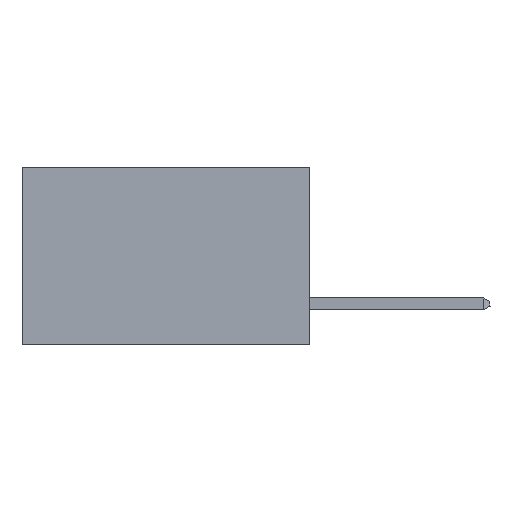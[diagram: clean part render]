
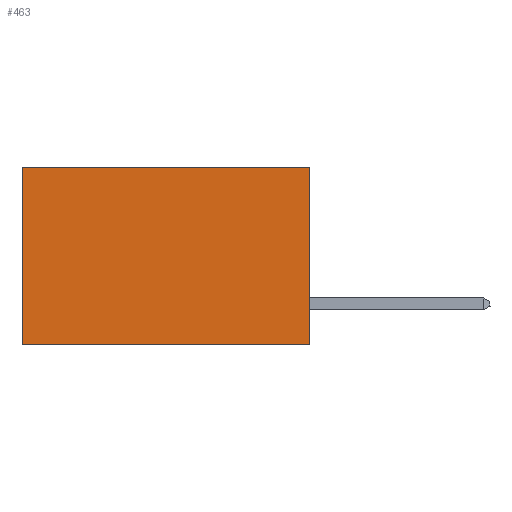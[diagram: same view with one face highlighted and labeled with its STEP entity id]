
A CAD part, left-side view. The second image highlights one B-rep face of the part: STEP entity #463.
In plain terms, the highlighted planar face has unit normal (-1, 0, 0).
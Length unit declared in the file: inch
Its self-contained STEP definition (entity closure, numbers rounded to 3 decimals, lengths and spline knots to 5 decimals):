
#463 = ADVANCED_FACE ( 'NONE', ( #3504 ), #22064, .F. ) ;
#1447 = CARTESIAN_POINT ( 'NONE',  ( 0.2875, 0., 0. ) ) ;
#1668 = ORIENTED_EDGE ( 'NONE', *, *, #17843, .T. ) ;
#1670 = LINE ( 'NONE', #1447, #18792 ) ;
#2592 = VERTEX_POINT ( 'NONE', #8639 ) ;
#2808 = LINE ( 'NONE', #9005, #14001 ) ;
#3261 = AXIS2_PLACEMENT_3D ( 'NONE', #5212, #9715, #4883 ) ;
#3504 = FACE_OUTER_BOUND ( 'NONE', #24174, .T. ) ;
#3709 = DIRECTION ( 'NONE',  ( 0., 0., -1. ) ) ;
#4883 = DIRECTION ( 'NONE',  ( 0., 0., -1. ) ) ;
#5212 = CARTESIAN_POINT ( 'NONE',  ( 0.2875, 0., 0. ) ) ;
#5467 = DIRECTION ( 'NONE',  ( 0., 0., -1. ) ) ;
#5626 = EDGE_CURVE ( 'NONE', #19287, #7444, #1670, .T. ) ;
#5739 = VERTEX_POINT ( 'NONE', #21953 ) ;
#7444 = VERTEX_POINT ( 'NONE', #19123 ) ;
#8464 = EDGE_CURVE ( 'NONE', #19287, #5739, #2808, .T. ) ;
#8639 = CARTESIAN_POINT ( 'NONE',  ( 0.2875, 0.6, -0.37 ) ) ;
#9005 = CARTESIAN_POINT ( 'NONE',  ( 0.2875, 0., 0. ) ) ;
#9715 = DIRECTION ( 'NONE',  ( 1., 0., 0. ) ) ;
#11364 = VECTOR ( 'NONE', #5467, 39.37008 ) ;
#12311 = ORIENTED_EDGE ( 'NONE', *, *, #8464, .T. ) ;
#14001 = VECTOR ( 'NONE', #15645, 39.37008 ) ;
#14217 = EDGE_CURVE ( 'NONE', #7444, #2592, #23059, .T. ) ;
#15355 = ORIENTED_EDGE ( 'NONE', *, *, #14217, .F. ) ;
#15645 = DIRECTION ( 'NONE',  ( 0., 1., 0. ) ) ;
#16422 = VECTOR ( 'NONE', #22245, 39.37008 ) ;
#17570 = ORIENTED_EDGE ( 'NONE', *, *, #5626, .F. ) ;
#17843 = EDGE_CURVE ( 'NONE', #5739, #2592, #17932, .T. ) ;
#17932 = LINE ( 'NONE', #23203, #11364 ) ;
#18792 = VECTOR ( 'NONE', #3709, 39.37008 ) ;
#19123 = CARTESIAN_POINT ( 'NONE',  ( 0.2875, 0., -0.37 ) ) ;
#19287 = VERTEX_POINT ( 'NONE', #23705 ) ;
#21953 = CARTESIAN_POINT ( 'NONE',  ( 0.2875, 0.6, 0. ) ) ;
#22064 = PLANE ( 'NONE',  #3261 ) ;
#22245 = DIRECTION ( 'NONE',  ( 0., 1., 0. ) ) ;
#23059 = LINE ( 'NONE', #24455, #16422 ) ;
#23203 = CARTESIAN_POINT ( 'NONE',  ( 0.2875, 0.6, 0. ) ) ;
#23705 = CARTESIAN_POINT ( 'NONE',  ( 0.2875, 0., 0. ) ) ;
#24174 = EDGE_LOOP ( 'NONE', ( #1668, #15355, #17570, #12311 ) ) ;
#24455 = CARTESIAN_POINT ( 'NONE',  ( 0.2875, 0., -0.37 ) ) ;
